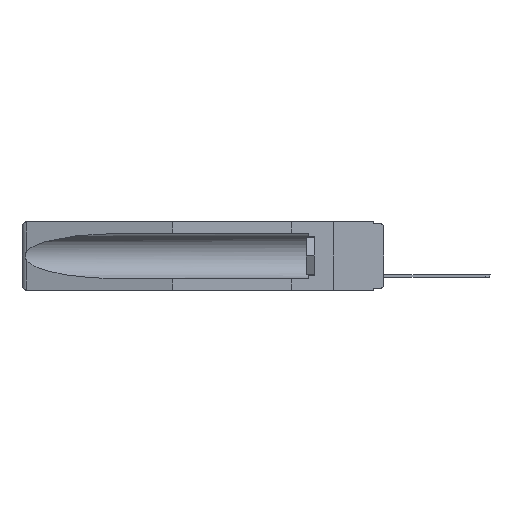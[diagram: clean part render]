
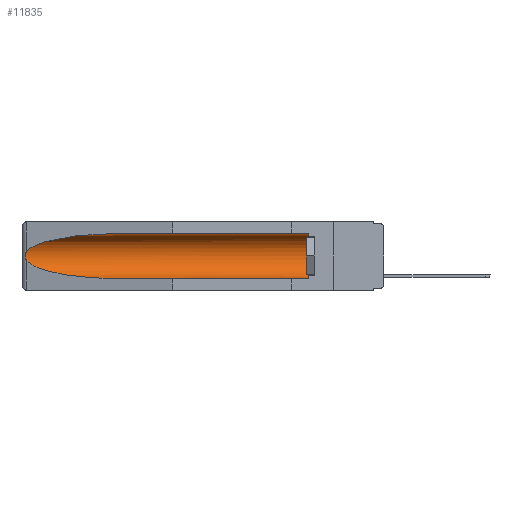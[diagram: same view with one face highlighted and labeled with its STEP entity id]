
A CAD part, left-side view. The second image highlights one B-rep face of the part: STEP entity #11835.
In plain terms, the highlighted cylindrical face has radius 2.857 mm (diameter 5.715 mm), a partial arc.
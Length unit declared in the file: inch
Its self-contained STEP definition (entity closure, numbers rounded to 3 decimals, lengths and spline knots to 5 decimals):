
#249 = VERTEX_POINT ( 'NONE', #9422 ) ;
#715 = VECTOR ( 'NONE', #15356, 39.37008 ) ;
#1171 = AXIS2_PLACEMENT_3D ( 'NONE', #19984, #10414, #10349 ) ;
#1716 = B_SPLINE_CURVE_WITH_KNOTS ( 'NONE', 3,
 ( #8749, #2675, #18795, #12432, #12360, #9327, #2822, #10706, #13713, #7916 ),
 .UNSPECIFIED., .F., .F.,
 ( 4, 2, 2, 2, 4 ),
 ( 0., 0.00029, 0.00058, 0.00087, 0.00117 ),
 .UNSPECIFIED. ) ;
#2462 = EDGE_CURVE ( 'NONE', #7762, #13809, #7398, .T. ) ;
#2675 = CARTESIAN_POINT ( 'NONE',  ( 0.26597, 1.52961, -0.15275 ) ) ;
#2822 = CARTESIAN_POINT ( 'NONE',  ( 0.2673, 1.53269, -0.17917 ) ) ;
#3580 = CARTESIAN_POINT ( 'NONE',  ( 0.155, 1.07973, -0.284 ) ) ;
#3595 = DIRECTION ( 'NONE',  ( 0., 0., 1. ) ) ;
#4030 = CARTESIAN_POINT ( 'NONE',  ( 0.26537, 1.52718, -0.14972 ) ) ;
#4133 = VECTOR ( 'NONE', #8309, 39.37008 ) ;
#5886 = ORIENTED_EDGE ( 'NONE', *, *, #6675, .T. ) ;
#6477 =( BOUNDED_CURVE ( )  B_SPLINE_CURVE ( 3, ( #20147, #13708, #15185, #4030 ),
 .UNSPECIFIED., .F., .F. ) 
 B_SPLINE_CURVE_WITH_KNOTS ( ( 4, 4 ),
 ( 4.71239, 6.08839 ),
 .UNSPECIFIED. ) 
 CURVE ( )  GEOMETRIC_REPRESENTATION_ITEM ( )  RATIONAL_B_SPLINE_CURVE ( ( 1., 0.848, 0.848, 1. ) ) 
 REPRESENTATION_ITEM ( '' )  );
#6675 = EDGE_CURVE ( 'NONE', #249, #7762, #1716, .T. ) ;
#7187 = CARTESIAN_POINT ( 'NONE',  ( 0.26537, 1.52718, -0.19328 ) ) ;
#7222 = AXIS2_PLACEMENT_3D ( 'NONE', #8396, #19572, #3595 ) ;
#7398 =( BOUNDED_CURVE ( )  B_SPLINE_CURVE ( 3, ( #7187, #8802, #18477, #14024 ),
 .UNSPECIFIED., .F., .T. ) 
 B_SPLINE_CURVE_WITH_KNOTS ( ( 4, 4 ),
 ( 0.1948, 1.5708 ),
 .UNSPECIFIED. ) 
 CURVE ( )  GEOMETRIC_REPRESENTATION_ITEM ( )  RATIONAL_B_SPLINE_CURVE ( ( 1., 0.848, 0.848, 1. ) ) 
 REPRESENTATION_ITEM ( '' )  );
#7762 = VERTEX_POINT ( 'NONE', #14000 ) ;
#7916 = CARTESIAN_POINT ( 'NONE',  ( 0.26537, 1.52718, -0.19328 ) ) ;
#8309 = DIRECTION ( 'NONE',  ( 0., 1., 0. ) ) ;
#8396 = CARTESIAN_POINT ( 'NONE',  ( 0.155, 0.126, -0.1715 ) ) ;
#8668 = ORIENTED_EDGE ( 'NONE', *, *, #2462, .T. ) ;
#8749 = CARTESIAN_POINT ( 'NONE',  ( 0.26537, 1.52718, -0.14972 ) ) ;
#8802 = CARTESIAN_POINT ( 'NONE',  ( 0.25451, 1.48313, -0.24835 ) ) ;
#9327 = CARTESIAN_POINT ( 'NONE',  ( 0.2675, 1.53308, -0.17534 ) ) ;
#9422 = CARTESIAN_POINT ( 'NONE',  ( 0.26537, 1.52718, -0.14972 ) ) ;
#9490 = EDGE_CURVE ( 'NONE', #10785, #12956, #17539, .T. ) ;
#9548 = ORIENTED_EDGE ( 'NONE', *, *, #20001, .T. ) ;
#9815 = ORIENTED_EDGE ( 'NONE', *, *, #20494, .F. ) ;
#10349 = DIRECTION ( 'NONE',  ( 0., 0., 1. ) ) ;
#10414 = DIRECTION ( 'NONE',  ( 0., 1., 0. ) ) ;
#10691 = CARTESIAN_POINT ( 'NONE',  ( 0.155, 0.126, -0.059 ) ) ;
#10706 = CARTESIAN_POINT ( 'NONE',  ( 0.26655, 1.53094, -0.18657 ) ) ;
#10785 = VERTEX_POINT ( 'NONE', #10691 ) ;
#11253 = EDGE_CURVE ( 'NONE', #12956, #249, #6477, .T. ) ;
#11835 = ADVANCED_FACE ( 'NONE', ( #16098 ), #17384, .F. ) ;
#12360 = CARTESIAN_POINT ( 'NONE',  ( 0.2675, 1.53308, -0.16763 ) ) ;
#12432 = CARTESIAN_POINT ( 'NONE',  ( 0.2673, 1.5327, -0.16383 ) ) ;
#12956 = VERTEX_POINT ( 'NONE', #19191 ) ;
#13708 = CARTESIAN_POINT ( 'NONE',  ( 0.21114, 1.30732, -0.059 ) ) ;
#13713 = CARTESIAN_POINT ( 'NONE',  ( 0.26597, 1.5296, -0.19026 ) ) ;
#13809 = VERTEX_POINT ( 'NONE', #3580 ) ;
#14000 = CARTESIAN_POINT ( 'NONE',  ( 0.26537, 1.52718, -0.19328 ) ) ;
#14024 = CARTESIAN_POINT ( 'NONE',  ( 0.155, 1.07973, -0.284 ) ) ;
#14339 = CARTESIAN_POINT ( 'NONE',  ( 0.155, 0.126, -0.284 ) ) ;
#14967 = ORIENTED_EDGE ( 'NONE', *, *, #11253, .T. ) ;
#14972 = VERTEX_POINT ( 'NONE', #14339 ) ;
#15185 = CARTESIAN_POINT ( 'NONE',  ( 0.25451, 1.48313, -0.09465 ) ) ;
#15356 = DIRECTION ( 'NONE',  ( 0., 1., 0. ) ) ;
#15971 = CIRCLE ( 'NONE', #7222, 0.1125 ) ;
#16098 = FACE_OUTER_BOUND ( 'NONE', #19017, .T. ) ;
#16441 = LINE ( 'NONE', #19485, #4133 ) ;
#17384 = CYLINDRICAL_SURFACE ( 'NONE', #1171, 0.1125 ) ;
#17539 = LINE ( 'NONE', #20474, #715 ) ;
#18477 = CARTESIAN_POINT ( 'NONE',  ( 0.21114, 1.30732, -0.284 ) ) ;
#18795 = CARTESIAN_POINT ( 'NONE',  ( 0.26654, 1.53092, -0.15636 ) ) ;
#19017 = EDGE_LOOP ( 'NONE', ( #14967, #5886, #8668, #9815, #9548, #20159 ) ) ;
#19191 = CARTESIAN_POINT ( 'NONE',  ( 0.155, 1.07973, -0.059 ) ) ;
#19485 = CARTESIAN_POINT ( 'NONE',  ( 0.155, -0.30754, -0.284 ) ) ;
#19572 = DIRECTION ( 'NONE',  ( 0., -1., 0. ) ) ;
#19984 = CARTESIAN_POINT ( 'NONE',  ( 0.155, -0.30754, -0.1715 ) ) ;
#20001 = EDGE_CURVE ( 'NONE', #14972, #10785, #15971, .T. ) ;
#20147 = CARTESIAN_POINT ( 'NONE',  ( 0.155, 1.07973, -0.059 ) ) ;
#20159 = ORIENTED_EDGE ( 'NONE', *, *, #9490, .T. ) ;
#20474 = CARTESIAN_POINT ( 'NONE',  ( 0.155, -0.30754, -0.059 ) ) ;
#20494 = EDGE_CURVE ( 'NONE', #14972, #13809, #16441, .T. ) ;
